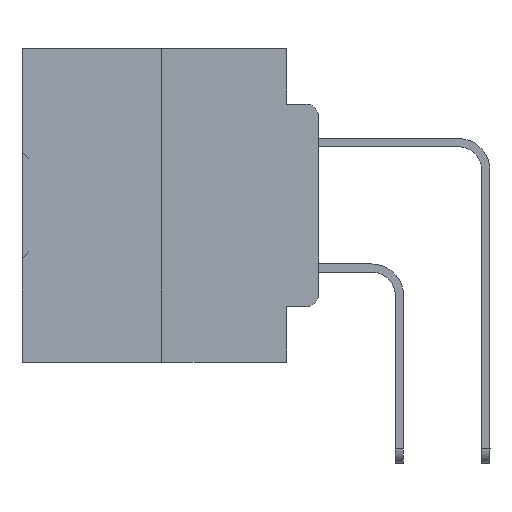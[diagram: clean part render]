
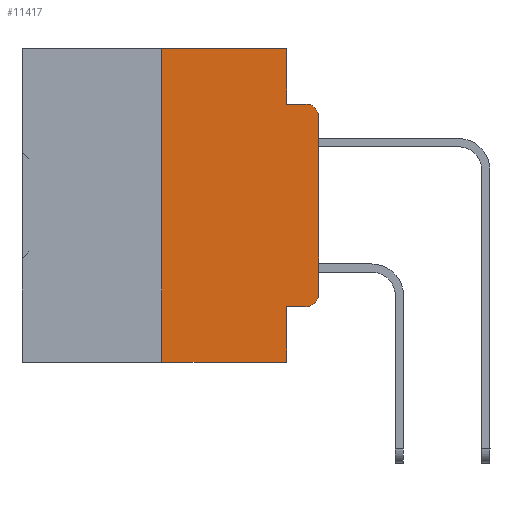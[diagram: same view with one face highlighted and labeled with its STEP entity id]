
A CAD part, left-side view. The second image highlights one B-rep face of the part: STEP entity #11417.
In plain terms, the highlighted planar face has unit normal (-1, 0, 0).
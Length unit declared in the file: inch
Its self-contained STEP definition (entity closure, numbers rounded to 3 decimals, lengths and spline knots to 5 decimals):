
#1304 = VERTEX_POINT ( 'NONE', #30322 ) ;
#1584 = DIRECTION ( 'NONE',  ( 0., 0., -1. ) ) ;
#3413 = LINE ( 'NONE', #32971, #16961 ) ;
#4074 = CIRCLE ( 'NONE', #8751, 0.02 ) ;
#4098 = EDGE_CURVE ( 'NONE', #27020, #34915, #4074, .T. ) ;
#4716 = CARTESIAN_POINT ( 'NONE',  ( 0., 0.051, -0.5 ) ) ;
#4957 = VERTEX_POINT ( 'NONE', #22455 ) ;
#5767 = DIRECTION ( 'NONE',  ( 1., 0., 0. ) ) ;
#6179 = EDGE_CURVE ( 'NONE', #39077, #34915, #21692, .T. ) ;
#6605 = ORIENTED_EDGE ( 'NONE', *, *, #27446, .T. ) ;
#6993 = VECTOR ( 'NONE', #9791, 39.37008 ) ;
#7109 = CARTESIAN_POINT ( 'NONE',  ( 0., 0.02, -0.1085 ) ) ;
#8346 = VECTOR ( 'NONE', #19631, 39.37008 ) ;
#8751 = AXIS2_PLACEMENT_3D ( 'NONE', #7109, #10052, #34770 ) ;
#8836 = VERTEX_POINT ( 'NONE', #4716 ) ;
#8924 = DIRECTION ( 'NONE',  ( 0., -1., 0. ) ) ;
#9054 = ORIENTED_EDGE ( 'NONE', *, *, #24885, .T. ) ;
#9234 = EDGE_LOOP ( 'NONE', ( #12175, #18874, #39202, #25919, #34071, #34515, #38461, #18991, #6605, #9054 ) ) ;
#9516 = CARTESIAN_POINT ( 'NONE',  ( 0., 0.051, -0.0885 ) ) ;
#9791 = DIRECTION ( 'NONE',  ( 0., -1., 0. ) ) ;
#10052 = DIRECTION ( 'NONE',  ( -1., 0., 0. ) ) ;
#11417 = ADVANCED_FACE ( 'NONE', ( #36891 ), #33684, .F. ) ;
#12175 = ORIENTED_EDGE ( 'NONE', *, *, #18901, .T. ) ;
#12357 = EDGE_CURVE ( 'NONE', #1304, #39077, #37242, .T. ) ;
#12579 = LINE ( 'NONE', #29711, #23255 ) ;
#12596 = CARTESIAN_POINT ( 'NONE',  ( 0., 0.051, -0.4115 ) ) ;
#13385 = VECTOR ( 'NONE', #8924, 39.37008 ) ;
#14772 = CARTESIAN_POINT ( 'NONE',  ( 0., 0.25, 0. ) ) ;
#15088 = VECTOR ( 'NONE', #19253, 39.37008 ) ;
#15425 = CARTESIAN_POINT ( 'NONE',  ( 0., 0.02, -0.0885 ) ) ;
#16241 = CARTESIAN_POINT ( 'NONE',  ( 0., 0.473, -0.5 ) ) ;
#16961 = VECTOR ( 'NONE', #17519, 39.37008 ) ;
#17332 = LINE ( 'NONE', #17957, #39015 ) ;
#17519 = DIRECTION ( 'NONE',  ( 0., 0., 1. ) ) ;
#17532 = CARTESIAN_POINT ( 'NONE',  ( 0., 0., 0. ) ) ;
#17957 = CARTESIAN_POINT ( 'NONE',  ( 0., 0.473, 0. ) ) ;
#18874 = ORIENTED_EDGE ( 'NONE', *, *, #4098, .T. ) ;
#18901 = EDGE_CURVE ( 'NONE', #4957, #27020, #30362, .T. ) ;
#18991 = ORIENTED_EDGE ( 'NONE', *, *, #30876, .F. ) ;
#19253 = DIRECTION ( 'NONE',  ( 0., 0., -1. ) ) ;
#19631 = DIRECTION ( 'NONE',  ( 0., -1., 0. ) ) ;
#21692 = LINE ( 'NONE', #30389, #13385 ) ;
#21896 = CARTESIAN_POINT ( 'NONE',  ( 0., 0.02, -0.3915 ) ) ;
#22182 = VECTOR ( 'NONE', #26668, 39.37008 ) ;
#22455 = CARTESIAN_POINT ( 'NONE',  ( 0., 0., -0.3915 ) ) ;
#22691 = AXIS2_PLACEMENT_3D ( 'NONE', #27110, #5767, #24143 ) ;
#23255 = VECTOR ( 'NONE', #1584, 39.37008 ) ;
#23706 = VERTEX_POINT ( 'NONE', #37413 ) ;
#24143 = DIRECTION ( 'NONE',  ( 0., 0., -1. ) ) ;
#24885 = EDGE_CURVE ( 'NONE', #31119, #4957, #26075, .T. ) ;
#25370 = LINE ( 'NONE', #28570, #6993 ) ;
#25919 = ORIENTED_EDGE ( 'NONE', *, *, #12357, .F. ) ;
#25973 = EDGE_CURVE ( 'NONE', #32136, #1304, #17332, .T. ) ;
#26075 = CIRCLE ( 'NONE', #35562, 0.02 ) ;
#26475 = CARTESIAN_POINT ( 'NONE',  ( 0., 0., -0.1085 ) ) ;
#26668 = DIRECTION ( 'NONE',  ( 0., 0., 1. ) ) ;
#27020 = VERTEX_POINT ( 'NONE', #26475 ) ;
#27110 = CARTESIAN_POINT ( 'NONE',  ( 0., 0.473, 0. ) ) ;
#27446 = EDGE_CURVE ( 'NONE', #27872, #31119, #25370, .T. ) ;
#27872 = VERTEX_POINT ( 'NONE', #12596 ) ;
#28182 = DIRECTION ( 'NONE',  ( 0., 0., -1. ) ) ;
#28570 = CARTESIAN_POINT ( 'NONE',  ( 0., 0.051, -0.4115 ) ) ;
#29243 = EDGE_CURVE ( 'NONE', #23706, #8836, #37272, .T. ) ;
#29711 = CARTESIAN_POINT ( 'NONE',  ( 0., 0.051, 0. ) ) ;
#30299 = EDGE_CURVE ( 'NONE', #23706, #32136, #3413, .T. ) ;
#30322 = CARTESIAN_POINT ( 'NONE',  ( 0., 0.051, 0. ) ) ;
#30362 = LINE ( 'NONE', #17532, #22182 ) ;
#30389 = CARTESIAN_POINT ( 'NONE',  ( 0., 0.051, -0.0885 ) ) ;
#30876 = EDGE_CURVE ( 'NONE', #27872, #8836, #12579, .T. ) ;
#31119 = VERTEX_POINT ( 'NONE', #36823 ) ;
#32136 = VERTEX_POINT ( 'NONE', #14772 ) ;
#32971 = CARTESIAN_POINT ( 'NONE',  ( 0., 0.25, 0. ) ) ;
#33144 = DIRECTION ( 'NONE',  ( 0., -1., 0. ) ) ;
#33684 = PLANE ( 'NONE',  #22691 ) ;
#34071 = ORIENTED_EDGE ( 'NONE', *, *, #25973, .F. ) ;
#34515 = ORIENTED_EDGE ( 'NONE', *, *, #30299, .F. ) ;
#34770 = DIRECTION ( 'NONE',  ( 0., 0., -1. ) ) ;
#34915 = VERTEX_POINT ( 'NONE', #15425 ) ;
#35562 = AXIS2_PLACEMENT_3D ( 'NONE', #21896, #37328, #28182 ) ;
#36823 = CARTESIAN_POINT ( 'NONE',  ( 0., 0.02, -0.4115 ) ) ;
#36891 = FACE_OUTER_BOUND ( 'NONE', #9234, .T. ) ;
#37242 = LINE ( 'NONE', #37691, #15088 ) ;
#37272 = LINE ( 'NONE', #16241, #8346 ) ;
#37328 = DIRECTION ( 'NONE',  ( -1., 0., 0. ) ) ;
#37413 = CARTESIAN_POINT ( 'NONE',  ( 0., 0.25, -0.5 ) ) ;
#37691 = CARTESIAN_POINT ( 'NONE',  ( 0., 0.051, 0. ) ) ;
#38461 = ORIENTED_EDGE ( 'NONE', *, *, #29243, .T. ) ;
#39015 = VECTOR ( 'NONE', #33144, 39.37008 ) ;
#39077 = VERTEX_POINT ( 'NONE', #9516 ) ;
#39202 = ORIENTED_EDGE ( 'NONE', *, *, #6179, .F. ) ;
